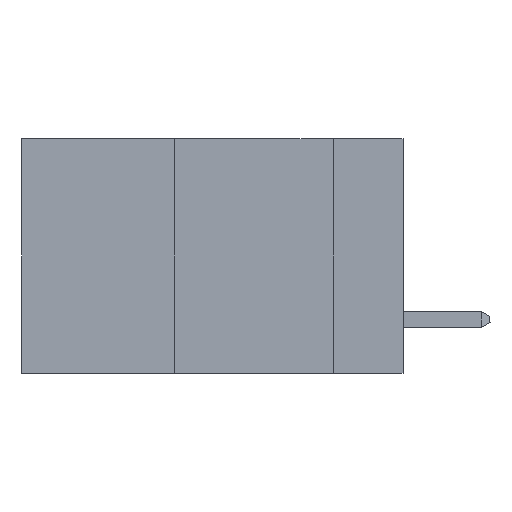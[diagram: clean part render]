
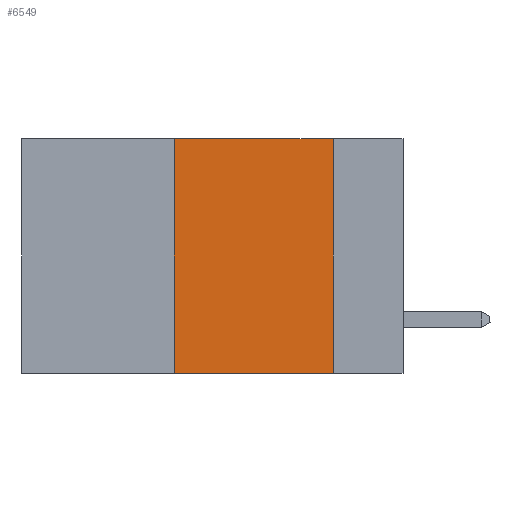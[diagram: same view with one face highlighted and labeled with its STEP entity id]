
A CAD part, left-side view. The second image highlights one B-rep face of the part: STEP entity #6549.
In plain terms, the highlighted planar face has unit normal (-1, 0, 0).
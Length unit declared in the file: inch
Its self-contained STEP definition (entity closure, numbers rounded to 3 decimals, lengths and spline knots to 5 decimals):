
#1572 = ORIENTED_EDGE ( 'NONE', *, *, #21562, .F. ) ;
#1703 = VECTOR ( 'NONE', #18859, 39.37008 ) ;
#1988 = DIRECTION ( 'NONE',  ( 1., 0., 0. ) ) ;
#4891 = CARTESIAN_POINT ( 'NONE',  ( 0., 0.36, 0. ) ) ;
#6501 = VERTEX_POINT ( 'NONE', #4891 ) ;
#6549 = ADVANCED_FACE ( 'NONE', ( #19961 ), #28190, .F. ) ;
#7084 = LINE ( 'NONE', #13082, #17582 ) ;
#7105 = ORIENTED_EDGE ( 'NONE', *, *, #15887, .T. ) ;
#8134 = LINE ( 'NONE', #11794, #1703 ) ;
#8358 = CARTESIAN_POINT ( 'NONE',  ( 0., 0.11, 0. ) ) ;
#9953 = DIRECTION ( 'NONE',  ( 0., 0., -1. ) ) ;
#11794 = CARTESIAN_POINT ( 'NONE',  ( 0., 0.6, -0.37 ) ) ;
#12183 = ORIENTED_EDGE ( 'NONE', *, *, #24511, .F. ) ;
#13082 = CARTESIAN_POINT ( 'NONE',  ( 0., 0.6, 0. ) ) ;
#13653 = LINE ( 'NONE', #17780, #29767 ) ;
#13662 = EDGE_LOOP ( 'NONE', ( #17113, #12183, #1572, #7105 ) ) ;
#14439 = VERTEX_POINT ( 'NONE', #17527 ) ;
#15887 = EDGE_CURVE ( 'NONE', #21800, #14439, #8134, .T. ) ;
#15920 = CARTESIAN_POINT ( 'NONE',  ( 0., 0.6, 0. ) ) ;
#16293 = VECTOR ( 'NONE', #22577, 39.37008 ) ;
#17113 = ORIENTED_EDGE ( 'NONE', *, *, #21528, .F. ) ;
#17122 = VERTEX_POINT ( 'NONE', #22840 ) ;
#17527 = CARTESIAN_POINT ( 'NONE',  ( 0., 0.11, -0.37 ) ) ;
#17582 = VECTOR ( 'NONE', #27812, 39.37008 ) ;
#17780 = CARTESIAN_POINT ( 'NONE',  ( 0., 0.36, 0. ) ) ;
#18859 = DIRECTION ( 'NONE',  ( 0., -1., 0. ) ) ;
#19961 = FACE_OUTER_BOUND ( 'NONE', #13662, .T. ) ;
#21528 = EDGE_CURVE ( 'NONE', #17122, #14439, #26764, .T. ) ;
#21562 = EDGE_CURVE ( 'NONE', #21800, #6501, #13653, .T. ) ;
#21800 = VERTEX_POINT ( 'NONE', #22353 ) ;
#22161 = AXIS2_PLACEMENT_3D ( 'NONE', #15920, #1988, #9953 ) ;
#22353 = CARTESIAN_POINT ( 'NONE',  ( 0., 0.36, -0.37 ) ) ;
#22577 = DIRECTION ( 'NONE',  ( 0., 0., -1. ) ) ;
#22840 = CARTESIAN_POINT ( 'NONE',  ( 0., 0.11, 0. ) ) ;
#24511 = EDGE_CURVE ( 'NONE', #6501, #17122, #7084, .T. ) ;
#26764 = LINE ( 'NONE', #8358, #16293 ) ;
#27812 = DIRECTION ( 'NONE',  ( 0., -1., 0. ) ) ;
#28190 = PLANE ( 'NONE',  #22161 ) ;
#29483 = DIRECTION ( 'NONE',  ( 0., 0., 1. ) ) ;
#29767 = VECTOR ( 'NONE', #29483, 39.37008 ) ;
